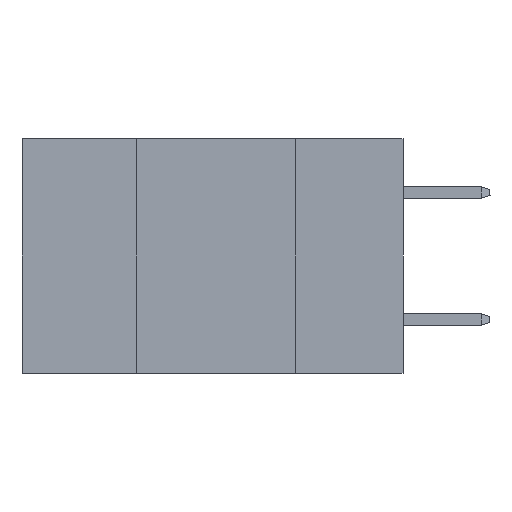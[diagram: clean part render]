
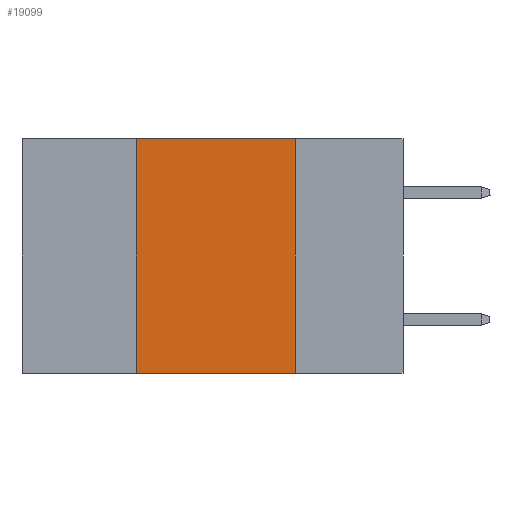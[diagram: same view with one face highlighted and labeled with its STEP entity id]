
A CAD part, left-side view. The second image highlights one B-rep face of the part: STEP entity #19099.
In plain terms, the highlighted planar face has unit normal (-1, 0, 0).
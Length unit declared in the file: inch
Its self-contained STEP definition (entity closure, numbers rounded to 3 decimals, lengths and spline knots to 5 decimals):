
#386 = CARTESIAN_POINT ( 'NONE',  ( 0., 0.6, 0. ) ) ;
#611 = VERTEX_POINT ( 'NONE', #27620 ) ;
#1023 = VECTOR ( 'NONE', #25412, 39.37008 ) ;
#1937 = VECTOR ( 'NONE', #17679, 39.37008 ) ;
#2374 = CARTESIAN_POINT ( 'NONE',  ( 0., 0.17, 0. ) ) ;
#2837 = EDGE_CURVE ( 'NONE', #43650, #31560, #24752, .T. ) ;
#3381 = LINE ( 'NONE', #7383, #1937 ) ;
#6492 = EDGE_LOOP ( 'NONE', ( #37333, #20605, #16888, #7127 ) ) ;
#7127 = ORIENTED_EDGE ( 'NONE', *, *, #18253, .T. ) ;
#7383 = CARTESIAN_POINT ( 'NONE',  ( 0., 0.6, -0.37 ) ) ;
#13135 = DIRECTION ( 'NONE',  ( 0., 0., -1. ) ) ;
#14037 = AXIS2_PLACEMENT_3D ( 'NONE', #386, #20292, #13135 ) ;
#14471 = DIRECTION ( 'NONE',  ( 0., 0., 1. ) ) ;
#14687 = CARTESIAN_POINT ( 'NONE',  ( 0., 0.42, 0. ) ) ;
#16888 = ORIENTED_EDGE ( 'NONE', *, *, #38952, .F. ) ;
#17679 = DIRECTION ( 'NONE',  ( 0., -1., 0. ) ) ;
#18253 = EDGE_CURVE ( 'NONE', #36398, #31560, #3381, .T. ) ;
#19099 = ADVANCED_FACE ( 'NONE', ( #41034 ), #31009, .F. ) ;
#20292 = DIRECTION ( 'NONE',  ( 1., 0., 0. ) ) ;
#20605 = ORIENTED_EDGE ( 'NONE', *, *, #42349, .F. ) ;
#21854 = LINE ( 'NONE', #14687, #26029 ) ;
#22672 = CARTESIAN_POINT ( 'NONE',  ( 0., 0.42, -0.37 ) ) ;
#23282 = VECTOR ( 'NONE', #37588, 39.37008 ) ;
#23996 = CARTESIAN_POINT ( 'NONE',  ( 0., 0.6, 0. ) ) ;
#24752 = LINE ( 'NONE', #2374, #1023 ) ;
#25412 = DIRECTION ( 'NONE',  ( 0., 0., -1. ) ) ;
#26029 = VECTOR ( 'NONE', #14471, 39.37008 ) ;
#27620 = CARTESIAN_POINT ( 'NONE',  ( 0., 0.42, 0. ) ) ;
#31009 = PLANE ( 'NONE',  #14037 ) ;
#31560 = VERTEX_POINT ( 'NONE', #31593 ) ;
#31593 = CARTESIAN_POINT ( 'NONE',  ( 0., 0.17, -0.37 ) ) ;
#34899 = CARTESIAN_POINT ( 'NONE',  ( 0., 0.17, 0. ) ) ;
#36398 = VERTEX_POINT ( 'NONE', #22672 ) ;
#37333 = ORIENTED_EDGE ( 'NONE', *, *, #2837, .F. ) ;
#37377 = LINE ( 'NONE', #23996, #23282 ) ;
#37588 = DIRECTION ( 'NONE',  ( 0., -1., 0. ) ) ;
#38952 = EDGE_CURVE ( 'NONE', #36398, #611, #21854, .T. ) ;
#41034 = FACE_OUTER_BOUND ( 'NONE', #6492, .T. ) ;
#42349 = EDGE_CURVE ( 'NONE', #611, #43650, #37377, .T. ) ;
#43650 = VERTEX_POINT ( 'NONE', #34899 ) ;
